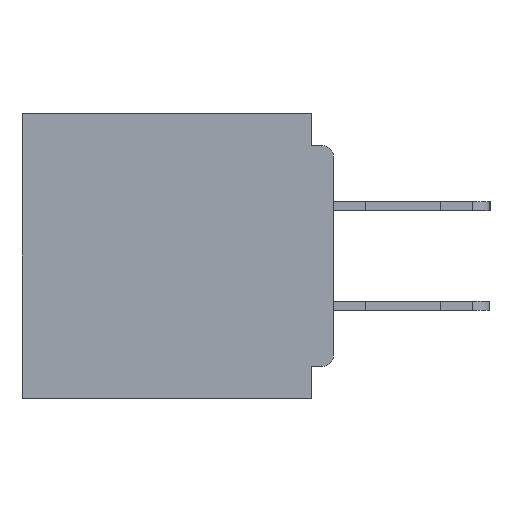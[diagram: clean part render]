
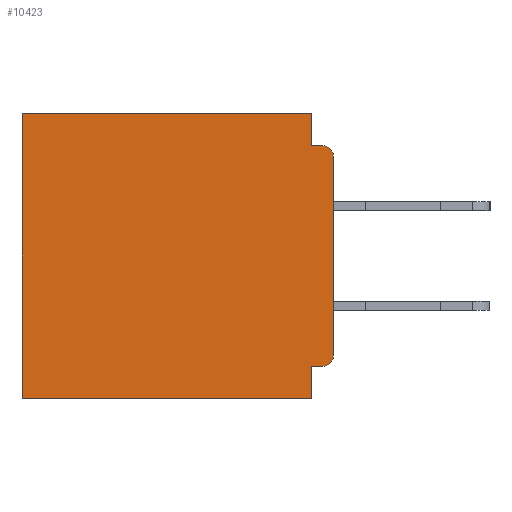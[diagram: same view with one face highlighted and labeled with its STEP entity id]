
A CAD part, left-side view. The second image highlights one B-rep face of the part: STEP entity #10423.
In plain terms, the highlighted planar face has unit normal (-1, 0, 0).
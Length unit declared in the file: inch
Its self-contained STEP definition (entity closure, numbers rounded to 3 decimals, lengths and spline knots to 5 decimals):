
#1066 = CARTESIAN_POINT ( 'NONE',  ( 0.3, 0., -0.355 ) ) ;
#1485 = VECTOR ( 'NONE', #4815, 39.37008 ) ;
#1806 = CARTESIAN_POINT ( 'NONE',  ( 0.3, 0.031, 0. ) ) ;
#2393 = AXIS2_PLACEMENT_3D ( 'NONE', #17110, #43788, #21018 ) ;
#2578 = VERTEX_POINT ( 'NONE', #13405 ) ;
#2822 = VECTOR ( 'NONE', #35316, 39.37008 ) ;
#2951 = ORIENTED_EDGE ( 'NONE', *, *, #47936, .F. ) ;
#3147 = CARTESIAN_POINT ( 'NONE',  ( 0.3, 0.015, -0.06 ) ) ;
#3584 = CARTESIAN_POINT ( 'NONE',  ( 0.3, 0., -0.4 ) ) ;
#3893 = ORIENTED_EDGE ( 'NONE', *, *, #11322, .F. ) ;
#4638 = CARTESIAN_POINT ( 'NONE',  ( 0.3, 0.031, 0. ) ) ;
#4694 = VERTEX_POINT ( 'NONE', #42765 ) ;
#4815 = DIRECTION ( 'NONE',  ( 0., 1., 0. ) ) ;
#5451 = LINE ( 'NONE', #12018, #23525 ) ;
#6393 = DIRECTION ( 'NONE',  ( 0., 0., -1. ) ) ;
#6519 = VECTOR ( 'NONE', #31491, 39.37008 ) ;
#6595 = VECTOR ( 'NONE', #6393, 39.37008 ) ;
#6781 = LINE ( 'NONE', #16389, #35001 ) ;
#6946 = DIRECTION ( 'NONE',  ( 0., 0., -1. ) ) ;
#7288 = EDGE_CURVE ( 'NONE', #35500, #12382, #5451, .T. ) ;
#7366 = DIRECTION ( 'NONE',  ( 0., 1., 0. ) ) ;
#7489 = LINE ( 'NONE', #12557, #47039 ) ;
#7712 = CARTESIAN_POINT ( 'NONE',  ( 0.3, 0.015, -0.34 ) ) ;
#8757 = VERTEX_POINT ( 'NONE', #1806 ) ;
#8789 = DIRECTION ( 'NONE',  ( 0., 1., 0. ) ) ;
#8865 = LINE ( 'NONE', #3584, #28126 ) ;
#9390 = AXIS2_PLACEMENT_3D ( 'NONE', #7712, #34597, #11564 ) ;
#9840 = VERTEX_POINT ( 'NONE', #43491 ) ;
#10155 = FACE_OUTER_BOUND ( 'NONE', #24322, .T. ) ;
#10423 = ADVANCED_FACE ( 'NONE', ( #10155 ), #32356, .F. ) ;
#10857 = ORIENTED_EDGE ( 'NONE', *, *, #45051, .T. ) ;
#10947 = ORIENTED_EDGE ( 'NONE', *, *, #36639, .F. ) ;
#11322 = EDGE_CURVE ( 'NONE', #9840, #14165, #8865, .T. ) ;
#11551 = LINE ( 'NONE', #1066, #1485 ) ;
#11564 = DIRECTION ( 'NONE',  ( 0., 0., -1. ) ) ;
#12018 = CARTESIAN_POINT ( 'NONE',  ( 0.3, 0., -0.045 ) ) ;
#12269 = EDGE_CURVE ( 'NONE', #45562, #9840, #12942, .T. ) ;
#12382 = VERTEX_POINT ( 'NONE', #17449 ) ;
#12557 = CARTESIAN_POINT ( 'NONE',  ( 0.3, 0.437, -0.4 ) ) ;
#12559 = EDGE_CURVE ( 'NONE', #41976, #12382, #40519, .T. ) ;
#12942 = LINE ( 'NONE', #31488, #2822 ) ;
#13405 = CARTESIAN_POINT ( 'NONE',  ( 0.3, 0.015, -0.355 ) ) ;
#13495 = ORIENTED_EDGE ( 'NONE', *, *, #12269, .F. ) ;
#13849 = ORIENTED_EDGE ( 'NONE', *, *, #46151, .T. ) ;
#14165 = VERTEX_POINT ( 'NONE', #15734 ) ;
#14951 = ORIENTED_EDGE ( 'NONE', *, *, #12559, .T. ) ;
#15734 = CARTESIAN_POINT ( 'NONE',  ( 0.3, 0.437, -0.4 ) ) ;
#15943 = DIRECTION ( 'NONE',  ( 0., -1., 0. ) ) ;
#16389 = CARTESIAN_POINT ( 'NONE',  ( 0.3, 0., 0. ) ) ;
#17110 = CARTESIAN_POINT ( 'NONE',  ( 0.3, 0., -0.4 ) ) ;
#17449 = CARTESIAN_POINT ( 'NONE',  ( 0.3, 0.015, -0.045 ) ) ;
#21018 = DIRECTION ( 'NONE',  ( 0., 0., -1. ) ) ;
#23525 = VECTOR ( 'NONE', #15943, 39.37008 ) ;
#24322 = EDGE_LOOP ( 'NONE', ( #2951, #14951, #43821, #10947, #13849, #10857, #3893, #13495, #27130, #45647 ) ) ;
#24479 = VERTEX_POINT ( 'NONE', #43484 ) ;
#26462 = CARTESIAN_POINT ( 'NONE',  ( 0.3, 0., -0.06 ) ) ;
#27066 = LINE ( 'NONE', #29429, #6595 ) ;
#27130 = ORIENTED_EDGE ( 'NONE', *, *, #41591, .F. ) ;
#27229 = AXIS2_PLACEMENT_3D ( 'NONE', #3147, #29984, #6946 ) ;
#27359 = CARTESIAN_POINT ( 'NONE',  ( 0.3, 0.031, -0.355 ) ) ;
#28126 = VECTOR ( 'NONE', #7366, 39.37008 ) ;
#29228 = EDGE_CURVE ( 'NONE', #2578, #4694, #42022, .T. ) ;
#29429 = CARTESIAN_POINT ( 'NONE',  ( 0.3, 0., -0.4 ) ) ;
#29984 = DIRECTION ( 'NONE',  ( -1., 0., 0. ) ) ;
#31488 = CARTESIAN_POINT ( 'NONE',  ( 0.3, 0.031, -0.4 ) ) ;
#31491 = DIRECTION ( 'NONE',  ( 0., 0., -1. ) ) ;
#32356 = PLANE ( 'NONE',  #2393 ) ;
#34597 = DIRECTION ( 'NONE',  ( -1., 0., 0. ) ) ;
#35001 = VECTOR ( 'NONE', #8789, 39.37008 ) ;
#35316 = DIRECTION ( 'NONE',  ( 0., 0., -1. ) ) ;
#35500 = VERTEX_POINT ( 'NONE', #47593 ) ;
#36639 = EDGE_CURVE ( 'NONE', #8757, #35500, #44866, .T. ) ;
#39571 = DIRECTION ( 'NONE',  ( 0., 0., -1. ) ) ;
#40519 = CIRCLE ( 'NONE', #27229, 0.015 ) ;
#41591 = EDGE_CURVE ( 'NONE', #2578, #45562, #11551, .T. ) ;
#41976 = VERTEX_POINT ( 'NONE', #26462 ) ;
#42022 = CIRCLE ( 'NONE', #9390, 0.015 ) ;
#42765 = CARTESIAN_POINT ( 'NONE',  ( 0.3, 0., -0.34 ) ) ;
#43484 = CARTESIAN_POINT ( 'NONE',  ( 0.3, 0.437, 0. ) ) ;
#43491 = CARTESIAN_POINT ( 'NONE',  ( 0.3, 0.031, -0.4 ) ) ;
#43788 = DIRECTION ( 'NONE',  ( 1., 0., 0. ) ) ;
#43821 = ORIENTED_EDGE ( 'NONE', *, *, #7288, .F. ) ;
#44866 = LINE ( 'NONE', #4638, #6519 ) ;
#45051 = EDGE_CURVE ( 'NONE', #24479, #14165, #7489, .T. ) ;
#45562 = VERTEX_POINT ( 'NONE', #27359 ) ;
#45647 = ORIENTED_EDGE ( 'NONE', *, *, #29228, .T. ) ;
#46151 = EDGE_CURVE ( 'NONE', #8757, #24479, #6781, .T. ) ;
#47039 = VECTOR ( 'NONE', #39571, 39.37008 ) ;
#47593 = CARTESIAN_POINT ( 'NONE',  ( 0.3, 0.031, -0.045 ) ) ;
#47936 = EDGE_CURVE ( 'NONE', #41976, #4694, #27066, .T. ) ;
